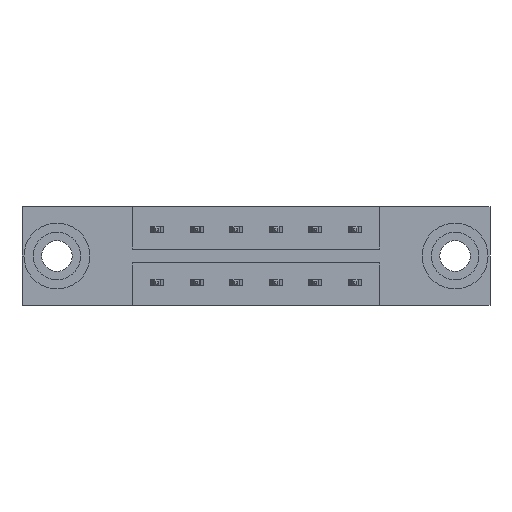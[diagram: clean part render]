
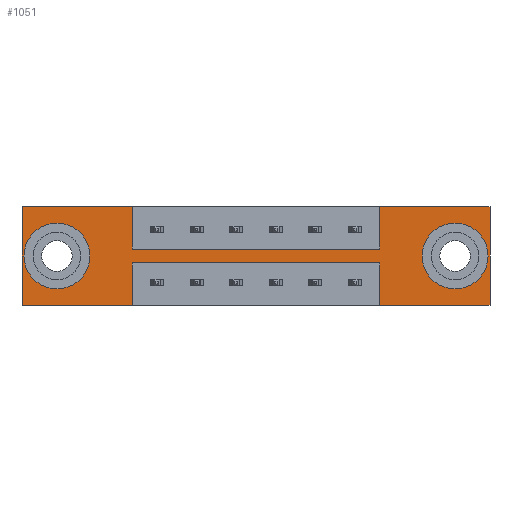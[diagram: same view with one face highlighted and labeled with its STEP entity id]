
A CAD part, front view. The second image highlights one B-rep face of the part: STEP entity #1051.
In plain terms, the highlighted planar face has unit normal (0, -1, 0).
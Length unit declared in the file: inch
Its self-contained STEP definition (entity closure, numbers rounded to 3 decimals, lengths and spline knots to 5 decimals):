
#54 = CARTESIAN_POINT ( 'NONE',  ( 1.775, 0., 0. ) ) ;
#74 = LINE ( 'NONE', #54, #1431 ) ;
#84 = ORIENTED_EDGE ( 'NONE', *, *, #1995, .T. ) ;
#135 = ORIENTED_EDGE ( 'NONE', *, *, #7400, .F. ) ;
#137 = EDGE_CURVE ( 'NONE', #2702, #3040, #4078, .T. ) ;
#176 = EDGE_CURVE ( 'NONE', #6181, #5695, #74, .T. ) ;
#182 = CARTESIAN_POINT ( 'NONE',  ( 1.3575, 0., -0.214 ) ) ;
#205 = EDGE_LOOP ( 'NONE', ( #6453, #5052 ) ) ;
#265 = CARTESIAN_POINT ( 'NONE',  ( 0., 0., 0. ) ) ;
#278 = CARTESIAN_POINT ( 'NONE',  ( 0., 0., -0.375 ) ) ;
#421 = EDGE_CURVE ( 'NONE', #7981, #7041, #5196, .T. ) ;
#471 = AXIS2_PLACEMENT_3D ( 'NONE', #3187, #5302, #3095 ) ;
#553 = ORIENTED_EDGE ( 'NONE', *, *, #8945, .F. ) ;
#587 = LINE ( 'NONE', #813, #8159 ) ;
#813 = CARTESIAN_POINT ( 'NONE',  ( 0.4175, 0., -0.214 ) ) ;
#818 = VERTEX_POINT ( 'NONE', #1001 ) ;
#897 = DIRECTION ( 'NONE',  ( -1., 0., 0. ) ) ;
#914 = CIRCLE ( 'NONE', #1027, 0.078 ) ;
#1001 = CARTESIAN_POINT ( 'NONE',  ( 1.6425, 0., -0.1095 ) ) ;
#1019 = DIRECTION ( 'NONE',  ( -1., 0., 0. ) ) ;
#1027 = AXIS2_PLACEMENT_3D ( 'NONE', #2002, #3940, #1841 ) ;
#1051 = ADVANCED_FACE ( 'NONE', ( #4619, #1077, #6425 ), #5291, .T. ) ;
#1077 = FACE_BOUND ( 'NONE', #205, .T. ) ;
#1105 = CARTESIAN_POINT ( 'NONE',  ( 0., 0., -0.375 ) ) ;
#1159 = CARTESIAN_POINT ( 'NONE',  ( 1.3575, 0., 0. ) ) ;
#1347 = CARTESIAN_POINT ( 'NONE',  ( 1.6425, 0., -0.1875 ) ) ;
#1363 = CARTESIAN_POINT ( 'NONE',  ( 1.775, 0., 0. ) ) ;
#1375 = CARTESIAN_POINT ( 'NONE',  ( 0., 0., 0. ) ) ;
#1429 = VERTEX_POINT ( 'NONE', #8525 ) ;
#1431 = VECTOR ( 'NONE', #5747, 39.37008 ) ;
#1549 = LINE ( 'NONE', #3088, #8875 ) ;
#1841 = DIRECTION ( 'NONE',  ( 0., 0., 1. ) ) ;
#1882 = EDGE_CURVE ( 'NONE', #8099, #818, #7273, .T. ) ;
#1960 = ORIENTED_EDGE ( 'NONE', *, *, #3924, .F. ) ;
#1995 = EDGE_CURVE ( 'NONE', #818, #8099, #4577, .T. ) ;
#2002 = CARTESIAN_POINT ( 'NONE',  ( 0.1325, 0., -0.1875 ) ) ;
#2058 = ORIENTED_EDGE ( 'NONE', *, *, #5631, .F. ) ;
#2164 = CARTESIAN_POINT ( 'NONE',  ( 1.6425, 0., -0.2655 ) ) ;
#2182 = DIRECTION ( 'NONE',  ( 1., 0., 0. ) ) ;
#2507 = VECTOR ( 'NONE', #2182, 39.37008 ) ;
#2509 = ORIENTED_EDGE ( 'NONE', *, *, #421, .F. ) ;
#2552 = VECTOR ( 'NONE', #1019, 39.37008 ) ;
#2621 = VECTOR ( 'NONE', #4923, 39.37008 ) ;
#2633 = VECTOR ( 'NONE', #6194, 39.37008 ) ;
#2645 = EDGE_CURVE ( 'NONE', #6700, #4920, #914, .T. ) ;
#2702 = VERTEX_POINT ( 'NONE', #4958 ) ;
#2716 = CARTESIAN_POINT ( 'NONE',  ( 0.4175, 0., -0.375 ) ) ;
#2978 = DIRECTION ( 'NONE',  ( 0., 0., 1. ) ) ;
#3040 = VERTEX_POINT ( 'NONE', #265 ) ;
#3088 = CARTESIAN_POINT ( 'NONE',  ( 1.3575, 0., -0.214 ) ) ;
#3095 = DIRECTION ( 'NONE',  ( 0., 0., 1. ) ) ;
#3164 = VECTOR ( 'NONE', #7944, 39.37008 ) ;
#3187 = CARTESIAN_POINT ( 'NONE',  ( 0.1325, 0., -0.1875 ) ) ;
#3213 = LINE ( 'NONE', #4401, #6794 ) ;
#3464 = ORIENTED_EDGE ( 'NONE', *, *, #3751, .F. ) ;
#3572 = ORIENTED_EDGE ( 'NONE', *, *, #4207, .F. ) ;
#3695 = EDGE_CURVE ( 'NONE', #6624, #2702, #3213, .T. ) ;
#3739 = EDGE_CURVE ( 'NONE', #4920, #6700, #4434, .T. ) ;
#3745 = CARTESIAN_POINT ( 'NONE',  ( 1.3575, 0., -0.161 ) ) ;
#3751 = EDGE_CURVE ( 'NONE', #5695, #4941, #6680, .T. ) ;
#3779 = CARTESIAN_POINT ( 'NONE',  ( 0.4175, 0., -0.214 ) ) ;
#3924 = EDGE_CURVE ( 'NONE', #7041, #7841, #4101, .T. ) ;
#3940 = DIRECTION ( 'NONE',  ( 0., 1., 0. ) ) ;
#4078 = LINE ( 'NONE', #8092, #4410 ) ;
#4097 = DIRECTION ( 'NONE',  ( 0., 1., 0. ) ) ;
#4101 = LINE ( 'NONE', #5526, #7456 ) ;
#4170 = VERTEX_POINT ( 'NONE', #182 ) ;
#4207 = EDGE_CURVE ( 'NONE', #4170, #1429, #8326, .T. ) ;
#4253 = EDGE_CURVE ( 'NONE', #4941, #4170, #1549, .T. ) ;
#4401 = CARTESIAN_POINT ( 'NONE',  ( 0., 0., -0.375 ) ) ;
#4410 = VECTOR ( 'NONE', #4535, 39.37008 ) ;
#4434 = CIRCLE ( 'NONE', #471, 0.078 ) ;
#4448 = CARTESIAN_POINT ( 'NONE',  ( 0.4175, 0., -0.161 ) ) ;
#4457 = DIRECTION ( 'NONE',  ( 0., -1., 0. ) ) ;
#4508 = LINE ( 'NONE', #1375, #2507 ) ;
#4535 = DIRECTION ( 'NONE',  ( 0., 0., 1. ) ) ;
#4577 = CIRCLE ( 'NONE', #6248, 0.078 ) ;
#4619 = FACE_BOUND ( 'NONE', #5305, .T. ) ;
#4694 = DIRECTION ( 'NONE',  ( 1., 0., 0. ) ) ;
#4805 = CARTESIAN_POINT ( 'NONE',  ( 0.4175, 0., -0.161 ) ) ;
#4823 = CARTESIAN_POINT ( 'NONE',  ( 0.4175, 0., 0. ) ) ;
#4907 = DIRECTION ( 'NONE',  ( 0., 0., -1. ) ) ;
#4920 = VERTEX_POINT ( 'NONE', #6617 ) ;
#4923 = DIRECTION ( 'NONE',  ( 1., 0., 0. ) ) ;
#4941 = VERTEX_POINT ( 'NONE', #5868 ) ;
#4958 = CARTESIAN_POINT ( 'NONE',  ( 0., 0., -0.375 ) ) ;
#5007 = ORIENTED_EDGE ( 'NONE', *, *, #4253, .F. ) ;
#5039 = CARTESIAN_POINT ( 'NONE',  ( 0., 0., 0. ) ) ;
#5052 = ORIENTED_EDGE ( 'NONE', *, *, #2645, .T. ) ;
#5061 = DIRECTION ( 'NONE',  ( 0., 0., -1. ) ) ;
#5098 = VECTOR ( 'NONE', #897, 39.37008 ) ;
#5196 = LINE ( 'NONE', #4805, #2633 ) ;
#5239 = VERTEX_POINT ( 'NONE', #1159 ) ;
#5255 = DIRECTION ( 'NONE',  ( 0., 0., -1. ) ) ;
#5291 = PLANE ( 'NONE',  #5658 ) ;
#5302 = DIRECTION ( 'NONE',  ( 0., 1., 0. ) ) ;
#5305 = EDGE_LOOP ( 'NONE', ( #84, #9016 ) ) ;
#5526 = CARTESIAN_POINT ( 'NONE',  ( 0.4175, 0., -0.161 ) ) ;
#5631 = EDGE_CURVE ( 'NONE', #7841, #5239, #6743, .T. ) ;
#5658 = AXIS2_PLACEMENT_3D ( 'NONE', #278, #4457, #5255 ) ;
#5695 = VERTEX_POINT ( 'NONE', #5883 ) ;
#5747 = DIRECTION ( 'NONE',  ( 0., 0., -1. ) ) ;
#5788 = ORIENTED_EDGE ( 'NONE', *, *, #137, .F. ) ;
#5863 = ORIENTED_EDGE ( 'NONE', *, *, #176, .F. ) ;
#5868 = CARTESIAN_POINT ( 'NONE',  ( 1.3575, 0., -0.375 ) ) ;
#5883 = CARTESIAN_POINT ( 'NONE',  ( 1.775, 0., -0.375 ) ) ;
#6075 = EDGE_LOOP ( 'NONE', ( #5007, #3464, #5863, #553, #2058, #1960, #2509, #6632, #5788, #7716, #135, #3572 ) ) ;
#6181 = VERTEX_POINT ( 'NONE', #1363 ) ;
#6182 = LINE ( 'NONE', #5039, #2621 ) ;
#6191 = DIRECTION ( 'NONE',  ( 0., 0., -1. ) ) ;
#6194 = DIRECTION ( 'NONE',  ( 0., 0., -1. ) ) ;
#6248 = AXIS2_PLACEMENT_3D ( 'NONE', #8354, #4097, #6191 ) ;
#6425 = FACE_OUTER_BOUND ( 'NONE', #6075, .T. ) ;
#6453 = ORIENTED_EDGE ( 'NONE', *, *, #3739, .T. ) ;
#6617 = CARTESIAN_POINT ( 'NONE',  ( 0.1325, 0., -0.1095 ) ) ;
#6624 = VERTEX_POINT ( 'NONE', #2716 ) ;
#6632 = ORIENTED_EDGE ( 'NONE', *, *, #8718, .F. ) ;
#6680 = LINE ( 'NONE', #1105, #2552 ) ;
#6700 = VERTEX_POINT ( 'NONE', #9082 ) ;
#6743 = LINE ( 'NONE', #3745, #3164 ) ;
#6794 = VECTOR ( 'NONE', #7216, 39.37008 ) ;
#7041 = VERTEX_POINT ( 'NONE', #4448 ) ;
#7216 = DIRECTION ( 'NONE',  ( -1., 0., 0. ) ) ;
#7273 = CIRCLE ( 'NONE', #8749, 0.078 ) ;
#7400 = EDGE_CURVE ( 'NONE', #1429, #6624, #587, .T. ) ;
#7456 = VECTOR ( 'NONE', #4694, 39.37008 ) ;
#7716 = ORIENTED_EDGE ( 'NONE', *, *, #3695, .F. ) ;
#7841 = VERTEX_POINT ( 'NONE', #8846 ) ;
#7944 = DIRECTION ( 'NONE',  ( 0., 0., 1. ) ) ;
#7981 = VERTEX_POINT ( 'NONE', #4823 ) ;
#8092 = CARTESIAN_POINT ( 'NONE',  ( 0., 0., 0. ) ) ;
#8099 = VERTEX_POINT ( 'NONE', #2164 ) ;
#8159 = VECTOR ( 'NONE', #5061, 39.37008 ) ;
#8326 = LINE ( 'NONE', #3779, #5098 ) ;
#8354 = CARTESIAN_POINT ( 'NONE',  ( 1.6425, 0., -0.1875 ) ) ;
#8525 = CARTESIAN_POINT ( 'NONE',  ( 0.4175, 0., -0.214 ) ) ;
#8718 = EDGE_CURVE ( 'NONE', #3040, #7981, #6182, .T. ) ;
#8749 = AXIS2_PLACEMENT_3D ( 'NONE', #1347, #9042, #4907 ) ;
#8846 = CARTESIAN_POINT ( 'NONE',  ( 1.3575, 0., -0.161 ) ) ;
#8875 = VECTOR ( 'NONE', #2978, 39.37008 ) ;
#8945 = EDGE_CURVE ( 'NONE', #5239, #6181, #4508, .T. ) ;
#9016 = ORIENTED_EDGE ( 'NONE', *, *, #1882, .T. ) ;
#9042 = DIRECTION ( 'NONE',  ( 0., 1., 0. ) ) ;
#9082 = CARTESIAN_POINT ( 'NONE',  ( 0.1325, 0., -0.2655 ) ) ;
